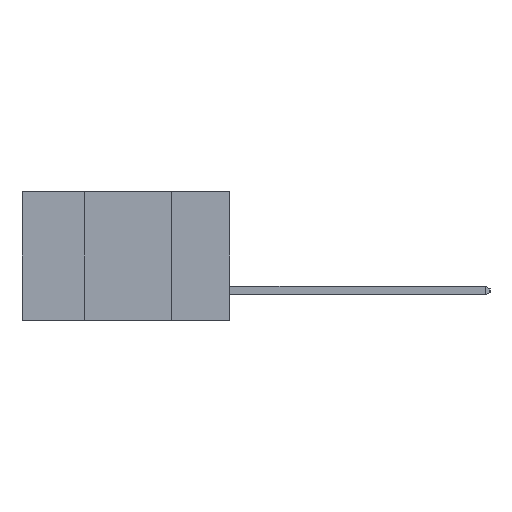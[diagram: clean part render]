
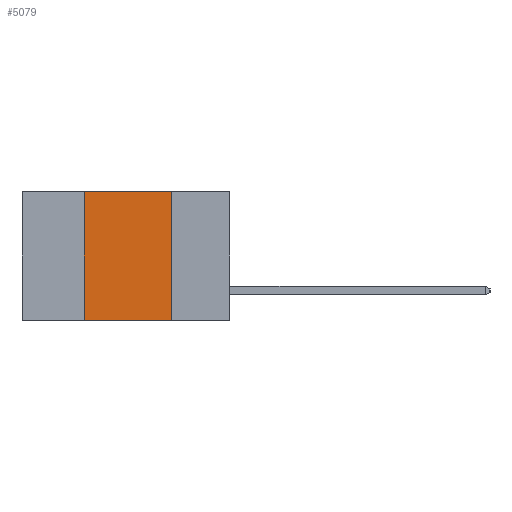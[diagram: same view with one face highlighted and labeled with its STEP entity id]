
A CAD part, left-side view. The second image highlights one B-rep face of the part: STEP entity #5079.
In plain terms, the highlighted planar face has unit normal (-1, 0, 0).
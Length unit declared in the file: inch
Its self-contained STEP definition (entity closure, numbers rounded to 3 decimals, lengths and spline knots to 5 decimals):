
#936 = ORIENTED_EDGE ( 'NONE', *, *, #20923, .T. ) ;
#2338 = CARTESIAN_POINT ( 'NONE',  ( 0., 0.6, -0.37 ) ) ;
#2576 = VERTEX_POINT ( 'NONE', #13709 ) ;
#4214 = CARTESIAN_POINT ( 'NONE',  ( 0., 0.42, 0. ) ) ;
#4389 = DIRECTION ( 'NONE',  ( 0., -1., 0. ) ) ;
#4955 = CARTESIAN_POINT ( 'NONE',  ( 0., 0.42, -0.37 ) ) ;
#5079 = ADVANCED_FACE ( 'NONE', ( #21766 ), #6069, .F. ) ;
#5441 = VECTOR ( 'NONE', #5856, 39.37008 ) ;
#5856 = DIRECTION ( 'NONE',  ( 0., 0., 1. ) ) ;
#6034 = DIRECTION ( 'NONE',  ( 0., 0., -1. ) ) ;
#6038 = DIRECTION ( 'NONE',  ( 1., 0., 0. ) ) ;
#6069 = PLANE ( 'NONE',  #9696 ) ;
#6213 = CARTESIAN_POINT ( 'NONE',  ( 0., 0.6, 0. ) ) ;
#8275 = ORIENTED_EDGE ( 'NONE', *, *, #9352, .F. ) ;
#9352 = EDGE_CURVE ( 'NONE', #19164, #23070, #18490, .T. ) ;
#9696 = AXIS2_PLACEMENT_3D ( 'NONE', #6213, #6038, #6034 ) ;
#13163 = VECTOR ( 'NONE', #16170, 39.37008 ) ;
#13709 = CARTESIAN_POINT ( 'NONE',  ( 0., 0.17, -0.37 ) ) ;
#15060 = LINE ( 'NONE', #18026, #5441 ) ;
#15571 = VERTEX_POINT ( 'NONE', #4955 ) ;
#15867 = CARTESIAN_POINT ( 'NONE',  ( 0., 0.6, 0. ) ) ;
#16170 = DIRECTION ( 'NONE',  ( 0., -1., 0. ) ) ;
#16339 = LINE ( 'NONE', #16439, #20997 ) ;
#16437 = LINE ( 'NONE', #2338, #25684 ) ;
#16439 = CARTESIAN_POINT ( 'NONE',  ( 0., 0.17, -0.37 ) ) ;
#18026 = CARTESIAN_POINT ( 'NONE',  ( 0., 0.42, -0.37 ) ) ;
#18102 = CARTESIAN_POINT ( 'NONE',  ( 0., 0.17, 0. ) ) ;
#18338 = DIRECTION ( 'NONE',  ( 0., 0., -1. ) ) ;
#18490 = LINE ( 'NONE', #15867, #13163 ) ;
#19164 = VERTEX_POINT ( 'NONE', #4214 ) ;
#20923 = EDGE_CURVE ( 'NONE', #15571, #2576, #16437, .T. ) ;
#20997 = VECTOR ( 'NONE', #18338, 39.37008 ) ;
#21766 = FACE_OUTER_BOUND ( 'NONE', #25747, .T. ) ;
#22137 = EDGE_CURVE ( 'NONE', #23070, #2576, #16339, .T. ) ;
#23037 = EDGE_CURVE ( 'NONE', #15571, #19164, #15060, .T. ) ;
#23040 = ORIENTED_EDGE ( 'NONE', *, *, #23037, .F. ) ;
#23070 = VERTEX_POINT ( 'NONE', #18102 ) ;
#24917 = ORIENTED_EDGE ( 'NONE', *, *, #22137, .F. ) ;
#25684 = VECTOR ( 'NONE', #4389, 39.37008 ) ;
#25747 = EDGE_LOOP ( 'NONE', ( #24917, #8275, #23040, #936 ) ) ;
